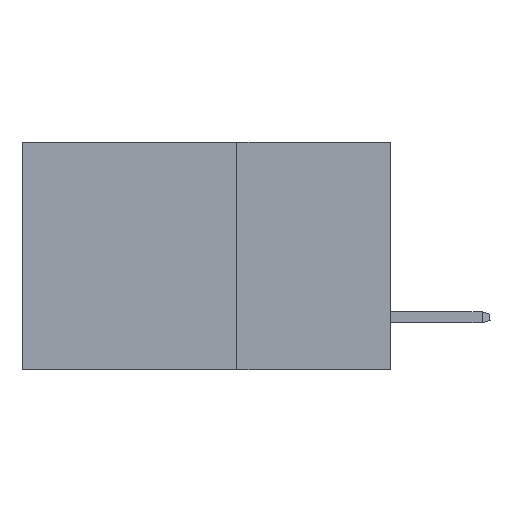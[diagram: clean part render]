
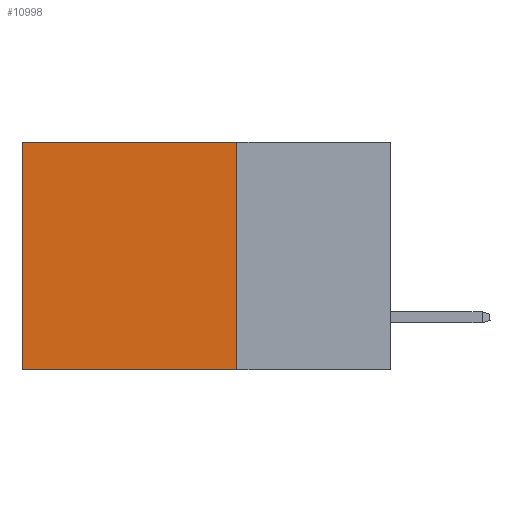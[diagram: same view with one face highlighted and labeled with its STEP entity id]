
A CAD part, left-side view. The second image highlights one B-rep face of the part: STEP entity #10998.
In plain terms, the highlighted planar face has unit normal (-1, 0, 0).
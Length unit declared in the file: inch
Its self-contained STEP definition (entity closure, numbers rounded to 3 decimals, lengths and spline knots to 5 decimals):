
#550 = LINE ( 'NONE', #8051, #19239 ) ;
#1384 = EDGE_CURVE ( 'NONE', #31104, #24557, #550, .T. ) ;
#2500 = DIRECTION ( 'NONE',  ( 0., 0., -1. ) ) ;
#8048 = VERTEX_POINT ( 'NONE', #10756 ) ;
#8051 = CARTESIAN_POINT ( 'NONE',  ( 0.2875, 0.25, -0.37 ) ) ;
#8387 = CARTESIAN_POINT ( 'NONE',  ( 0.2875, 0.6, 0. ) ) ;
#10151 = AXIS2_PLACEMENT_3D ( 'NONE', #14454, #35974, #2500 ) ;
#10756 = CARTESIAN_POINT ( 'NONE',  ( 0.2875, 0.6, 0. ) ) ;
#10998 = ADVANCED_FACE ( 'NONE', ( #17635 ), #33048, .F. ) ;
#12106 = EDGE_LOOP ( 'NONE', ( #22621, #12644, #31430, #34321 ) ) ;
#12631 = VECTOR ( 'NONE', #17328, 39.37008 ) ;
#12644 = ORIENTED_EDGE ( 'NONE', *, *, #1384, .F. ) ;
#14454 = CARTESIAN_POINT ( 'NONE',  ( 0.2875, 0.25, 0. ) ) ;
#14576 = CARTESIAN_POINT ( 'NONE',  ( 0.2875, 0.6, -0.37 ) ) ;
#16201 = DIRECTION ( 'NONE',  ( 0., 0., -1. ) ) ;
#17328 = DIRECTION ( 'NONE',  ( 0., 1., 0. ) ) ;
#17359 = EDGE_CURVE ( 'NONE', #26582, #31104, #24577, .T. ) ;
#17635 = FACE_OUTER_BOUND ( 'NONE', #12106, .T. ) ;
#19239 = VECTOR ( 'NONE', #23360, 39.37008 ) ;
#19582 = CARTESIAN_POINT ( 'NONE',  ( 0.2875, 0.25, 0. ) ) ;
#19760 = VECTOR ( 'NONE', #33073, 39.37008 ) ;
#21232 = EDGE_CURVE ( 'NONE', #8048, #24557, #27944, .T. ) ;
#22621 = ORIENTED_EDGE ( 'NONE', *, *, #21232, .T. ) ;
#23360 = DIRECTION ( 'NONE',  ( 0., 1., 0. ) ) ;
#24557 = VERTEX_POINT ( 'NONE', #14576 ) ;
#24577 = LINE ( 'NONE', #19582, #33236 ) ;
#26582 = VERTEX_POINT ( 'NONE', #39085 ) ;
#27944 = LINE ( 'NONE', #8387, #19760 ) ;
#29154 = EDGE_CURVE ( 'NONE', #26582, #8048, #36660, .T. ) ;
#31104 = VERTEX_POINT ( 'NONE', #37713 ) ;
#31430 = ORIENTED_EDGE ( 'NONE', *, *, #17359, .F. ) ;
#32791 = CARTESIAN_POINT ( 'NONE',  ( 0.2875, 0.25, 0. ) ) ;
#33048 = PLANE ( 'NONE',  #10151 ) ;
#33073 = DIRECTION ( 'NONE',  ( 0., 0., -1. ) ) ;
#33236 = VECTOR ( 'NONE', #16201, 39.37008 ) ;
#34321 = ORIENTED_EDGE ( 'NONE', *, *, #29154, .T. ) ;
#35974 = DIRECTION ( 'NONE',  ( 1., 0., 0. ) ) ;
#36660 = LINE ( 'NONE', #32791, #12631 ) ;
#37713 = CARTESIAN_POINT ( 'NONE',  ( 0.2875, 0.25, -0.37 ) ) ;
#39085 = CARTESIAN_POINT ( 'NONE',  ( 0.2875, 0.25, 0. ) ) ;
